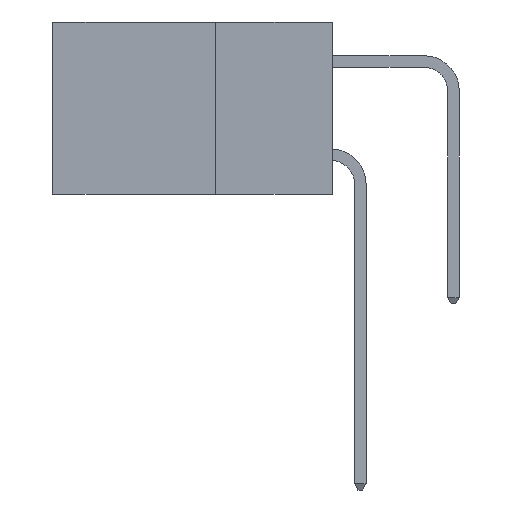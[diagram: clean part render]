
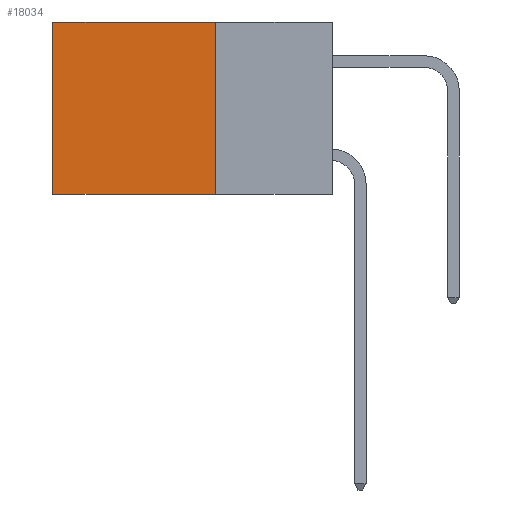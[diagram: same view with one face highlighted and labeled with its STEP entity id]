
A CAD part, left-side view. The second image highlights one B-rep face of the part: STEP entity #18034.
In plain terms, the highlighted planar face has unit normal (-1, 0, 0).
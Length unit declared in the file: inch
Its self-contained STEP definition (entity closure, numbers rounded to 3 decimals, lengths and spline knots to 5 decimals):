
#485 = EDGE_LOOP ( 'NONE', ( #19290, #7431, #6177, #17993 ) ) ;
#1040 = EDGE_CURVE ( 'NONE', #3285, #17202, #7559, .T. ) ;
#2248 = DIRECTION ( 'NONE',  ( 0., 0., -1. ) ) ;
#3285 = VERTEX_POINT ( 'NONE', #3612 ) ;
#3612 = CARTESIAN_POINT ( 'NONE',  ( 0.2615, 0.25, -0.37 ) ) ;
#4417 = DIRECTION ( 'NONE',  ( 1., 0., 0. ) ) ;
#4644 = CARTESIAN_POINT ( 'NONE',  ( 0.2615, 0.25, 0. ) ) ;
#4885 = CARTESIAN_POINT ( 'NONE',  ( 0.2615, 0.25, 0. ) ) ;
#6060 = AXIS2_PLACEMENT_3D ( 'NONE', #13525, #4417, #15053 ) ;
#6177 = ORIENTED_EDGE ( 'NONE', *, *, #15096, .F. ) ;
#6587 = EDGE_CURVE ( 'NONE', #6757, #17202, #8553, .T. ) ;
#6757 = VERTEX_POINT ( 'NONE', #9984 ) ;
#6914 = VERTEX_POINT ( 'NONE', #4885 ) ;
#7431 = ORIENTED_EDGE ( 'NONE', *, *, #1040, .F. ) ;
#7559 = LINE ( 'NONE', #12702, #18187 ) ;
#8006 = CARTESIAN_POINT ( 'NONE',  ( 0.2615, 0.6, -0.37 ) ) ;
#8553 = LINE ( 'NONE', #14002, #16153 ) ;
#8770 = DIRECTION ( 'NONE',  ( 0., 1., 0. ) ) ;
#9756 = LINE ( 'NONE', #4644, #13794 ) ;
#9810 = CARTESIAN_POINT ( 'NONE',  ( 0.2615, 0.25, -0.37 ) ) ;
#9984 = CARTESIAN_POINT ( 'NONE',  ( 0.2615, 0.6, 0. ) ) ;
#11158 = VECTOR ( 'NONE', #2248, 39.37008 ) ;
#11638 = LINE ( 'NONE', #9810, #11158 ) ;
#12230 = DIRECTION ( 'NONE',  ( 0., 1., 0. ) ) ;
#12702 = CARTESIAN_POINT ( 'NONE',  ( 0.2615, 0.25, -0.37 ) ) ;
#13525 = CARTESIAN_POINT ( 'NONE',  ( 0.2615, 0.25, -0.37 ) ) ;
#13794 = VECTOR ( 'NONE', #12230, 39.37008 ) ;
#13980 = DIRECTION ( 'NONE',  ( 0., 0., -1. ) ) ;
#14002 = CARTESIAN_POINT ( 'NONE',  ( 0.2615, 0.6, -0.37 ) ) ;
#15053 = DIRECTION ( 'NONE',  ( 0., 0., -1. ) ) ;
#15096 = EDGE_CURVE ( 'NONE', #6914, #3285, #11638, .T. ) ;
#16153 = VECTOR ( 'NONE', #13980, 39.37008 ) ;
#17037 = EDGE_CURVE ( 'NONE', #6914, #6757, #9756, .T. ) ;
#17202 = VERTEX_POINT ( 'NONE', #8006 ) ;
#17521 = FACE_OUTER_BOUND ( 'NONE', #485, .T. ) ;
#17993 = ORIENTED_EDGE ( 'NONE', *, *, #17037, .T. ) ;
#18034 = ADVANCED_FACE ( 'NONE', ( #17521 ), #19466, .F. ) ;
#18187 = VECTOR ( 'NONE', #8770, 39.37008 ) ;
#19290 = ORIENTED_EDGE ( 'NONE', *, *, #6587, .T. ) ;
#19466 = PLANE ( 'NONE',  #6060 ) ;
